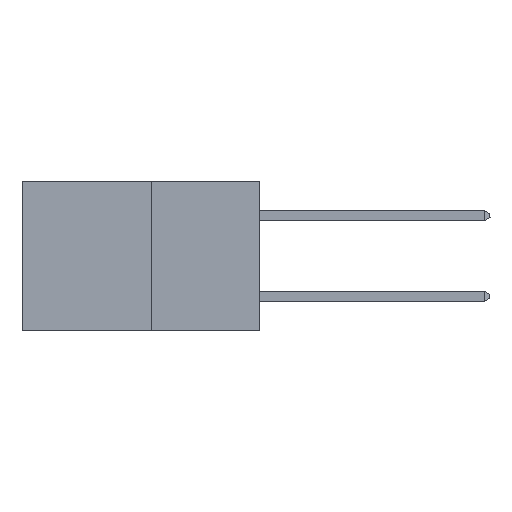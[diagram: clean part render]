
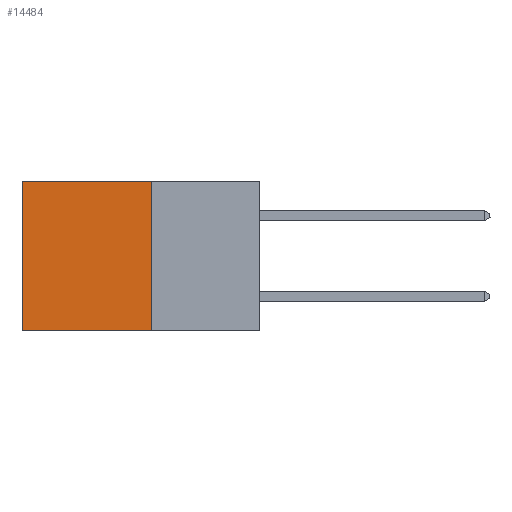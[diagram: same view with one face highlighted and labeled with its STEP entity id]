
A CAD part, left-side view. The second image highlights one B-rep face of the part: STEP entity #14484.
In plain terms, the highlighted planar face has unit normal (-1, 0, 0).
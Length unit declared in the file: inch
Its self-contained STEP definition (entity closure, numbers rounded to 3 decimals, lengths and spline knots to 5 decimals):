
#312 = LINE ( 'NONE', #1745, #17031 ) ;
#330 = ORIENTED_EDGE ( 'NONE', *, *, #7884, .T. ) ;
#795 = VERTEX_POINT ( 'NONE', #3422 ) ;
#1233 = VERTEX_POINT ( 'NONE', #17725 ) ;
#1745 = CARTESIAN_POINT ( 'NONE',  ( 0.277, 0.59, -0.37 ) ) ;
#1766 = DIRECTION ( 'NONE',  ( 0., 1., 0. ) ) ;
#2219 = EDGE_CURVE ( 'NONE', #795, #1233, #7266, .T. ) ;
#2679 = DIRECTION ( 'NONE',  ( 0., 1., 0. ) ) ;
#3422 = CARTESIAN_POINT ( 'NONE',  ( 0.277, 0.27, 0. ) ) ;
#4015 = EDGE_CURVE ( 'NONE', #8503, #8519, #312, .T. ) ;
#4392 = ORIENTED_EDGE ( 'NONE', *, *, #19413, .F. ) ;
#5286 = AXIS2_PLACEMENT_3D ( 'NONE', #20743, #15994, #6358 ) ;
#5428 = ORIENTED_EDGE ( 'NONE', *, *, #4015, .T. ) ;
#6358 = DIRECTION ( 'NONE',  ( 0., 0., -1. ) ) ;
#7266 = LINE ( 'NONE', #17197, #19591 ) ;
#7277 = EDGE_LOOP ( 'NONE', ( #5428, #4392, #12306, #330 ) ) ;
#7884 = EDGE_CURVE ( 'NONE', #795, #8503, #11472, .T. ) ;
#8503 = VERTEX_POINT ( 'NONE', #16158 ) ;
#8519 = VERTEX_POINT ( 'NONE', #9697 ) ;
#9502 = DIRECTION ( 'NONE',  ( 0., 0., -1. ) ) ;
#9697 = CARTESIAN_POINT ( 'NONE',  ( 0.277, 0.59, -0.37 ) ) ;
#10193 = FACE_OUTER_BOUND ( 'NONE', #7277, .T. ) ;
#10708 = CARTESIAN_POINT ( 'NONE',  ( 0.277, 0.27, -0.37 ) ) ;
#11457 = LINE ( 'NONE', #10708, #20006 ) ;
#11472 = LINE ( 'NONE', #19489, #15245 ) ;
#12306 = ORIENTED_EDGE ( 'NONE', *, *, #2219, .F. ) ;
#14381 = PLANE ( 'NONE',  #5286 ) ;
#14484 = ADVANCED_FACE ( 'NONE', ( #10193 ), #14381, .F. ) ;
#15245 = VECTOR ( 'NONE', #1766, 39.37008 ) ;
#15994 = DIRECTION ( 'NONE',  ( 1., 0., 0. ) ) ;
#16158 = CARTESIAN_POINT ( 'NONE',  ( 0.277, 0.59, 0. ) ) ;
#16313 = DIRECTION ( 'NONE',  ( 0., 0., -1. ) ) ;
#17031 = VECTOR ( 'NONE', #16313, 39.37008 ) ;
#17197 = CARTESIAN_POINT ( 'NONE',  ( 0.277, 0.27, -0.37 ) ) ;
#17725 = CARTESIAN_POINT ( 'NONE',  ( 0.277, 0.27, -0.37 ) ) ;
#19413 = EDGE_CURVE ( 'NONE', #1233, #8519, #11457, .T. ) ;
#19489 = CARTESIAN_POINT ( 'NONE',  ( 0.277, 0.27, 0. ) ) ;
#19591 = VECTOR ( 'NONE', #9502, 39.37008 ) ;
#20006 = VECTOR ( 'NONE', #2679, 39.37008 ) ;
#20743 = CARTESIAN_POINT ( 'NONE',  ( 0.277, 0.27, -0.37 ) ) ;
